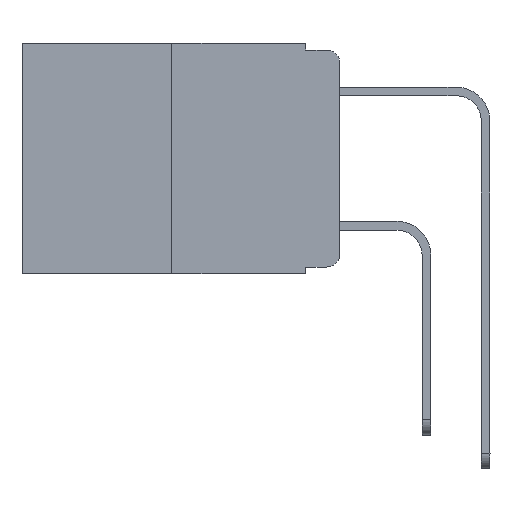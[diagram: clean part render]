
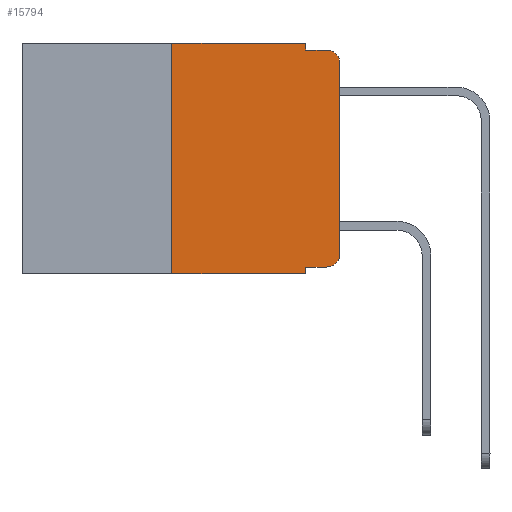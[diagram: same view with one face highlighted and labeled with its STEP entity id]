
A CAD part, left-side view. The second image highlights one B-rep face of the part: STEP entity #15794.
In plain terms, the highlighted planar face has unit normal (-1, 0, 0).
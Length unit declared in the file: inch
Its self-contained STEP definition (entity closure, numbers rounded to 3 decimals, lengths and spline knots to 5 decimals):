
#365 = CARTESIAN_POINT ( 'NONE',  ( 0., 0.473, -0.343 ) ) ;
#412 = ORIENTED_EDGE ( 'NONE', *, *, #13065, .T. ) ;
#1173 = DIRECTION ( 'NONE',  ( 0., -1., 0. ) ) ;
#1366 = CARTESIAN_POINT ( 'NONE',  ( 0., 0., -0.313 ) ) ;
#1427 = CARTESIAN_POINT ( 'NONE',  ( 0., 0.473, 0. ) ) ;
#1670 = CARTESIAN_POINT ( 'NONE',  ( 0., 0.051, -0.01 ) ) ;
#1714 = VERTEX_POINT ( 'NONE', #8028 ) ;
#1717 = CARTESIAN_POINT ( 'NONE',  ( 0., 0.051, 0. ) ) ;
#2178 = LINE ( 'NONE', #365, #20611 ) ;
#2338 = VECTOR ( 'NONE', #11048, 39.37008 ) ;
#2771 = VERTEX_POINT ( 'NONE', #9248 ) ;
#2828 = EDGE_CURVE ( 'NONE', #3893, #21241, #23511, .T. ) ;
#3161 = DIRECTION ( 'NONE',  ( 0., 0., -1. ) ) ;
#3893 = VERTEX_POINT ( 'NONE', #24547 ) ;
#4182 = EDGE_CURVE ( 'NONE', #4449, #5640, #2178, .T. ) ;
#4390 = ORIENTED_EDGE ( 'NONE', *, *, #4182, .T. ) ;
#4449 = VERTEX_POINT ( 'NONE', #18778 ) ;
#4473 = AXIS2_PLACEMENT_3D ( 'NONE', #15873, #5825, #21643 ) ;
#5080 = CARTESIAN_POINT ( 'NONE',  ( 0., 0.051, -0.333 ) ) ;
#5182 = CARTESIAN_POINT ( 'NONE',  ( 0., 0.051, -0.343 ) ) ;
#5292 = CARTESIAN_POINT ( 'NONE',  ( 0., 0.051, -0.01 ) ) ;
#5312 = EDGE_CURVE ( 'NONE', #16426, #18138, #5960, .T. ) ;
#5640 = VERTEX_POINT ( 'NONE', #5182 ) ;
#5739 = CIRCLE ( 'NONE', #4473, 0.02 ) ;
#5825 = DIRECTION ( 'NONE',  ( -1., 0., 0. ) ) ;
#5860 = CARTESIAN_POINT ( 'NONE',  ( 0., 0.473, 0. ) ) ;
#5960 = CIRCLE ( 'NONE', #14269, 0.02 ) ;
#6630 = ORIENTED_EDGE ( 'NONE', *, *, #6735, .F. ) ;
#6659 = CARTESIAN_POINT ( 'NONE',  ( 0., 0.02, -0.333 ) ) ;
#6735 = EDGE_CURVE ( 'NONE', #15525, #5640, #21584, .T. ) ;
#7145 = LINE ( 'NONE', #13532, #2338 ) ;
#7236 = EDGE_LOOP ( 'NONE', ( #12155, #412, #19561, #25151, #21629, #15104, #4390, #6630, #17855, #19303 ) ) ;
#8028 = CARTESIAN_POINT ( 'NONE',  ( 0., 0.02, -0.01 ) ) ;
#9248 = CARTESIAN_POINT ( 'NONE',  ( 0., 0., -0.03 ) ) ;
#9499 = DIRECTION ( 'NONE',  ( 1., 0., 0. ) ) ;
#10129 = DIRECTION ( 'NONE',  ( 0., -1., 0. ) ) ;
#10161 = CARTESIAN_POINT ( 'NONE',  ( 0., 0.051, -0.333 ) ) ;
#10318 = CARTESIAN_POINT ( 'NONE',  ( 0., 0.02, -0.313 ) ) ;
#10447 = DIRECTION ( 'NONE',  ( 0., 0., 1. ) ) ;
#10701 = EDGE_CURVE ( 'NONE', #18138, #2771, #7145, .T. ) ;
#11048 = DIRECTION ( 'NONE',  ( 0., 0., 1. ) ) ;
#11053 = LINE ( 'NONE', #1427, #23416 ) ;
#12155 = ORIENTED_EDGE ( 'NONE', *, *, #10701, .T. ) ;
#12643 = EDGE_CURVE ( 'NONE', #15525, #16426, #21144, .T. ) ;
#12736 = VECTOR ( 'NONE', #25329, 39.37008 ) ;
#13044 = VECTOR ( 'NONE', #10447, 39.37008 ) ;
#13065 = EDGE_CURVE ( 'NONE', #2771, #1714, #5739, .T. ) ;
#13532 = CARTESIAN_POINT ( 'NONE',  ( 0., 0., 0. ) ) ;
#14269 = AXIS2_PLACEMENT_3D ( 'NONE', #10318, #18306, #24582 ) ;
#15104 = ORIENTED_EDGE ( 'NONE', *, *, #19548, .F. ) ;
#15515 = FACE_OUTER_BOUND ( 'NONE', #7236, .T. ) ;
#15525 = VERTEX_POINT ( 'NONE', #10161 ) ;
#15794 = ADVANCED_FACE ( 'NONE', ( #15515 ), #21806, .F. ) ;
#15873 = CARTESIAN_POINT ( 'NONE',  ( 0., 0.02, -0.03 ) ) ;
#16335 = LINE ( 'NONE', #24327, #13044 ) ;
#16362 = CARTESIAN_POINT ( 'NONE',  ( 0., 0.25, 0. ) ) ;
#16426 = VERTEX_POINT ( 'NONE', #6659 ) ;
#17033 = EDGE_CURVE ( 'NONE', #22792, #3893, #11053, .T. ) ;
#17093 = CARTESIAN_POINT ( 'NONE',  ( 0., 0.051, 0. ) ) ;
#17479 = DIRECTION ( 'NONE',  ( 0., 0., -1. ) ) ;
#17855 = ORIENTED_EDGE ( 'NONE', *, *, #12643, .T. ) ;
#18138 = VERTEX_POINT ( 'NONE', #1366 ) ;
#18306 = DIRECTION ( 'NONE',  ( -1., 0., 0. ) ) ;
#18778 = CARTESIAN_POINT ( 'NONE',  ( 0., 0.25, -0.343 ) ) ;
#19072 = VECTOR ( 'NONE', #1173, 39.37008 ) ;
#19303 = ORIENTED_EDGE ( 'NONE', *, *, #5312, .T. ) ;
#19548 = EDGE_CURVE ( 'NONE', #4449, #22792, #16335, .T. ) ;
#19561 = ORIENTED_EDGE ( 'NONE', *, *, #25362, .F. ) ;
#19566 = LINE ( 'NONE', #1670, #25480 ) ;
#20436 = AXIS2_PLACEMENT_3D ( 'NONE', #5860, #9499, #17479 ) ;
#20611 = VECTOR ( 'NONE', #10129, 39.37008 ) ;
#21141 = DIRECTION ( 'NONE',  ( 0., -1., 0. ) ) ;
#21144 = LINE ( 'NONE', #5080, #19072 ) ;
#21241 = VERTEX_POINT ( 'NONE', #5292 ) ;
#21584 = LINE ( 'NONE', #1717, #23249 ) ;
#21629 = ORIENTED_EDGE ( 'NONE', *, *, #17033, .F. ) ;
#21643 = DIRECTION ( 'NONE',  ( 0., 0., -1. ) ) ;
#21806 = PLANE ( 'NONE',  #20436 ) ;
#22792 = VERTEX_POINT ( 'NONE', #16362 ) ;
#23249 = VECTOR ( 'NONE', #3161, 39.37008 ) ;
#23360 = DIRECTION ( 'NONE',  ( 0., -1., 0. ) ) ;
#23416 = VECTOR ( 'NONE', #21141, 39.37008 ) ;
#23511 = LINE ( 'NONE', #17093, #12736 ) ;
#24327 = CARTESIAN_POINT ( 'NONE',  ( 0., 0.25, 0. ) ) ;
#24547 = CARTESIAN_POINT ( 'NONE',  ( 0., 0.051, 0. ) ) ;
#24582 = DIRECTION ( 'NONE',  ( 0., 0., -1. ) ) ;
#25151 = ORIENTED_EDGE ( 'NONE', *, *, #2828, .F. ) ;
#25329 = DIRECTION ( 'NONE',  ( 0., 0., -1. ) ) ;
#25362 = EDGE_CURVE ( 'NONE', #21241, #1714, #19566, .T. ) ;
#25480 = VECTOR ( 'NONE', #23360, 39.37008 ) ;
